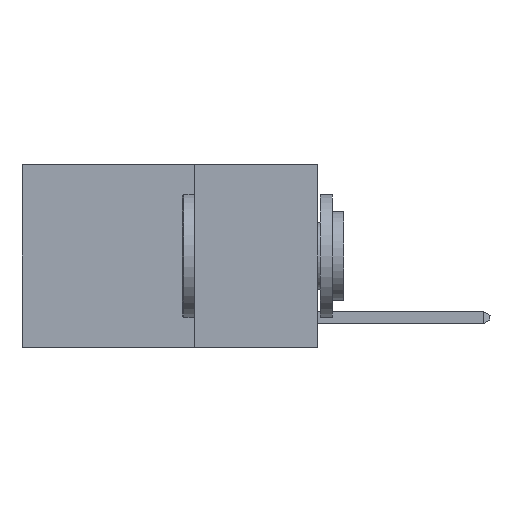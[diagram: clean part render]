
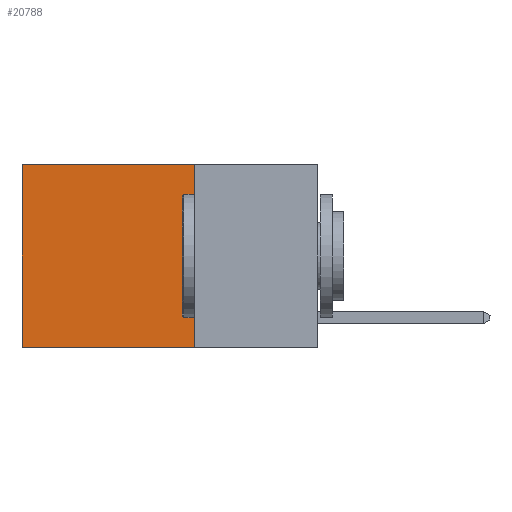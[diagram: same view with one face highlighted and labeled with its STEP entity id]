
A CAD part, left-side view. The second image highlights one B-rep face of the part: STEP entity #20788.
In plain terms, the highlighted planar face has unit normal (-1, 0, 0).
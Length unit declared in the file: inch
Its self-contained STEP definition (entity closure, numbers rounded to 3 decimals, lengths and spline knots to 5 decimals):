
#532 = CARTESIAN_POINT ( 'NONE',  ( 0.2625, 0.6, 0. ) ) ;
#723 = CARTESIAN_POINT ( 'NONE',  ( 0.2625, 0.6, 0. ) ) ;
#1183 = VECTOR ( 'NONE', #22110, 39.37008 ) ;
#1207 = FACE_OUTER_BOUND ( 'NONE', #7804, .T. ) ;
#2499 = CARTESIAN_POINT ( 'NONE',  ( 0.2625, 0.25, 0. ) ) ;
#3891 = VERTEX_POINT ( 'NONE', #9973 ) ;
#4728 = LINE ( 'NONE', #723, #16458 ) ;
#4877 = AXIS2_PLACEMENT_3D ( 'NONE', #10923, #20503, #18583 ) ;
#5205 = DIRECTION ( 'NONE',  ( 0., 1., 0. ) ) ;
#6777 = CARTESIAN_POINT ( 'NONE',  ( 0.2625, 0.25, 0. ) ) ;
#7224 = VERTEX_POINT ( 'NONE', #532 ) ;
#7334 = VERTEX_POINT ( 'NONE', #2499 ) ;
#7804 = EDGE_LOOP ( 'NONE', ( #16455, #24621, #15393, #9766 ) ) ;
#9016 = CARTESIAN_POINT ( 'NONE',  ( 0.2625, 0.25, -0.37 ) ) ;
#9488 = CARTESIAN_POINT ( 'NONE',  ( 0.2625, 0.25, -0.37 ) ) ;
#9524 = LINE ( 'NONE', #9488, #14659 ) ;
#9766 = ORIENTED_EDGE ( 'NONE', *, *, #12845, .T. ) ;
#9973 = CARTESIAN_POINT ( 'NONE',  ( 0.2625, 0.6, -0.37 ) ) ;
#10923 = CARTESIAN_POINT ( 'NONE',  ( 0.2625, 0.25, 0. ) ) ;
#11506 = VECTOR ( 'NONE', #13067, 39.37008 ) ;
#12017 = EDGE_CURVE ( 'NONE', #7224, #3891, #4728, .T. ) ;
#12845 = EDGE_CURVE ( 'NONE', #7334, #7224, #14280, .T. ) ;
#13067 = DIRECTION ( 'NONE',  ( 0., 1., 0. ) ) ;
#14280 = LINE ( 'NONE', #20662, #11506 ) ;
#14659 = VECTOR ( 'NONE', #5205, 39.37008 ) ;
#15393 = ORIENTED_EDGE ( 'NONE', *, *, #18993, .F. ) ;
#16455 = ORIENTED_EDGE ( 'NONE', *, *, #12017, .T. ) ;
#16458 = VECTOR ( 'NONE', #21572, 39.37008 ) ;
#18455 = EDGE_CURVE ( 'NONE', #19752, #3891, #9524, .T. ) ;
#18583 = DIRECTION ( 'NONE',  ( 0., 0., -1. ) ) ;
#18888 = LINE ( 'NONE', #6777, #1183 ) ;
#18993 = EDGE_CURVE ( 'NONE', #7334, #19752, #18888, .T. ) ;
#19752 = VERTEX_POINT ( 'NONE', #9016 ) ;
#20503 = DIRECTION ( 'NONE',  ( 1., 0., 0. ) ) ;
#20556 = PLANE ( 'NONE',  #4877 ) ;
#20662 = CARTESIAN_POINT ( 'NONE',  ( 0.2625, 0.25, 0. ) ) ;
#20788 = ADVANCED_FACE ( 'NONE', ( #1207 ), #20556, .F. ) ;
#21572 = DIRECTION ( 'NONE',  ( 0., 0., -1. ) ) ;
#22110 = DIRECTION ( 'NONE',  ( 0., 0., -1. ) ) ;
#24621 = ORIENTED_EDGE ( 'NONE', *, *, #18455, .F. ) ;
